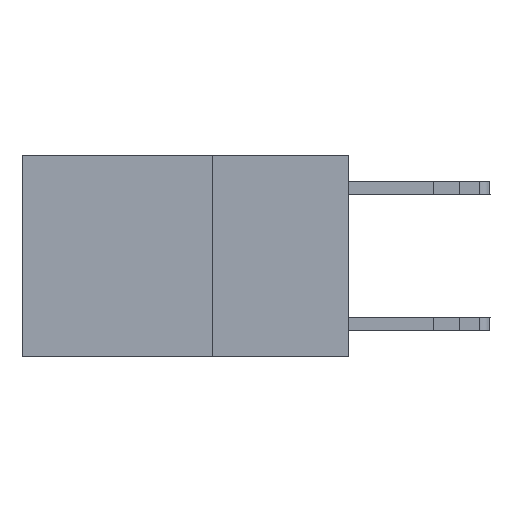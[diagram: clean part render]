
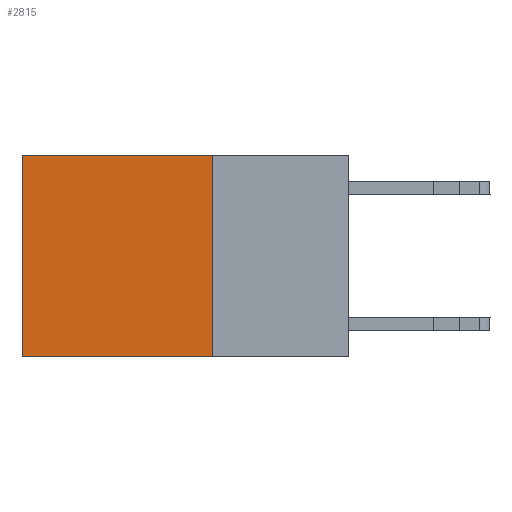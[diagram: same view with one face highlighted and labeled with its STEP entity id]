
A CAD part, left-side view. The second image highlights one B-rep face of the part: STEP entity #2815.
In plain terms, the highlighted planar face has unit normal (-1, 0, 0).
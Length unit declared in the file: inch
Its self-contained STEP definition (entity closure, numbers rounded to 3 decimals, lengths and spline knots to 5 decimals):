
#127 = EDGE_CURVE ( 'NONE', #2766, #10662, #6202, .T. ) ;
#153 = PLANE ( 'NONE',  #732 ) ;
#405 = CARTESIAN_POINT ( 'NONE',  ( 0.2625, 0.25, -0.37 ) ) ;
#732 = AXIS2_PLACEMENT_3D ( 'NONE', #2094, #10943, #937 ) ;
#806 = LINE ( 'NONE', #4775, #2229 ) ;
#937 = DIRECTION ( 'NONE',  ( 0., 0., -1. ) ) ;
#979 = CARTESIAN_POINT ( 'NONE',  ( 0.2625, 0.25, 0. ) ) ;
#1307 = DIRECTION ( 'NONE',  ( 0., 1., 0. ) ) ;
#1493 = ORIENTED_EDGE ( 'NONE', *, *, #2936, .F. ) ;
#2031 = FACE_OUTER_BOUND ( 'NONE', #4505, .T. ) ;
#2094 = CARTESIAN_POINT ( 'NONE',  ( 0.2625, 0.25, 0. ) ) ;
#2136 = CARTESIAN_POINT ( 'NONE',  ( 0.2625, 0.6, -0.37 ) ) ;
#2160 = ORIENTED_EDGE ( 'NONE', *, *, #2281, .T. ) ;
#2229 = VECTOR ( 'NONE', #12637, 39.37008 ) ;
#2281 = EDGE_CURVE ( 'NONE', #8147, #10662, #806, .T. ) ;
#2385 = VECTOR ( 'NONE', #2931, 39.37008 ) ;
#2766 = VERTEX_POINT ( 'NONE', #405 ) ;
#2791 = VECTOR ( 'NONE', #9655, 39.37008 ) ;
#2815 = ADVANCED_FACE ( 'NONE', ( #2031 ), #153, .F. ) ;
#2848 = ORIENTED_EDGE ( 'NONE', *, *, #12003, .T. ) ;
#2931 = DIRECTION ( 'NONE',  ( 0., 1., 0. ) ) ;
#2936 = EDGE_CURVE ( 'NONE', #4206, #2766, #5720, .T. ) ;
#3098 = VECTOR ( 'NONE', #1307, 39.37008 ) ;
#3845 = CARTESIAN_POINT ( 'NONE',  ( 0.2625, 0.25, 0. ) ) ;
#4043 = CARTESIAN_POINT ( 'NONE',  ( 0.2625, 0.25, -0.37 ) ) ;
#4179 = CARTESIAN_POINT ( 'NONE',  ( 0.2625, 0.6, 0. ) ) ;
#4206 = VERTEX_POINT ( 'NONE', #12355 ) ;
#4505 = EDGE_LOOP ( 'NONE', ( #2160, #7955, #1493, #2848 ) ) ;
#4775 = CARTESIAN_POINT ( 'NONE',  ( 0.2625, 0.6, 0. ) ) ;
#5720 = LINE ( 'NONE', #979, #2791 ) ;
#6202 = LINE ( 'NONE', #4043, #3098 ) ;
#7955 = ORIENTED_EDGE ( 'NONE', *, *, #127, .F. ) ;
#8147 = VERTEX_POINT ( 'NONE', #4179 ) ;
#9655 = DIRECTION ( 'NONE',  ( 0., 0., -1. ) ) ;
#10662 = VERTEX_POINT ( 'NONE', #2136 ) ;
#10943 = DIRECTION ( 'NONE',  ( 1., 0., 0. ) ) ;
#11980 = LINE ( 'NONE', #3845, #2385 ) ;
#12003 = EDGE_CURVE ( 'NONE', #4206, #8147, #11980, .T. ) ;
#12355 = CARTESIAN_POINT ( 'NONE',  ( 0.2625, 0.25, 0. ) ) ;
#12637 = DIRECTION ( 'NONE',  ( 0., 0., -1. ) ) ;
